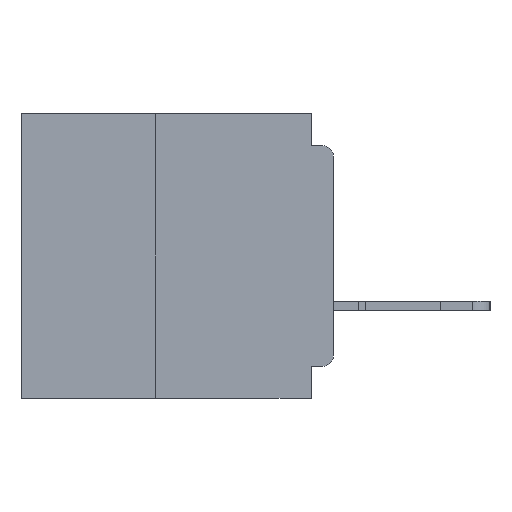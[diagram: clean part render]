
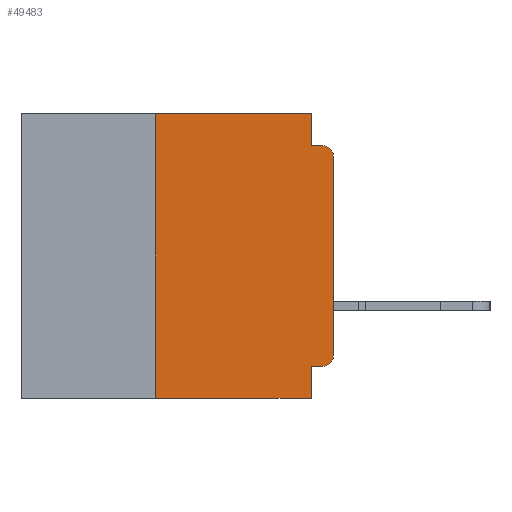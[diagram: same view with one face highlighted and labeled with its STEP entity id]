
A CAD part, left-side view. The second image highlights one B-rep face of the part: STEP entity #49483.
In plain terms, the highlighted planar face has unit normal (-1, 0, 0).
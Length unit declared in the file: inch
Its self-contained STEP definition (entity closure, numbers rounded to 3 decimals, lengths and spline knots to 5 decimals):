
#467 = DIRECTION ( 'NONE',  ( 0., 1., 0. ) ) ;
#2096 = CARTESIAN_POINT ( 'NONE',  ( 0., 0.25, -0.4 ) ) ;
#3207 = EDGE_LOOP ( 'NONE', ( #60867, #43556, #61168, #53774, #62017, #53021, #16379, #43665, #39169, #30989 ) ) ;
#4250 = VECTOR ( 'NONE', #64130, 39.37008 ) ;
#5299 = VERTEX_POINT ( 'NONE', #43062 ) ;
#7291 = LINE ( 'NONE', #30291, #57075 ) ;
#7347 = DIRECTION ( 'NONE',  ( 0., 0., -1. ) ) ;
#8504 = DIRECTION ( 'NONE',  ( 0., -1., 0. ) ) ;
#10152 = CARTESIAN_POINT ( 'NONE',  ( 0., 0.031, 0. ) ) ;
#11619 = EDGE_CURVE ( 'NONE', #15801, #20066, #23603, .T. ) ;
#11772 = VERTEX_POINT ( 'NONE', #50795 ) ;
#12141 = DIRECTION ( 'NONE',  ( 0., 0., 1. ) ) ;
#15801 = VERTEX_POINT ( 'NONE', #27613 ) ;
#15934 = VECTOR ( 'NONE', #12141, 39.37008 ) ;
#16250 = VECTOR ( 'NONE', #8504, 39.37008 ) ;
#16379 = ORIENTED_EDGE ( 'NONE', *, *, #63830, .T. ) ;
#17343 = VERTEX_POINT ( 'NONE', #45705 ) ;
#17473 = LINE ( 'NONE', #39353, #4250 ) ;
#18425 = VERTEX_POINT ( 'NONE', #45819 ) ;
#20066 = VERTEX_POINT ( 'NONE', #33617 ) ;
#20998 = CARTESIAN_POINT ( 'NONE',  ( 0., 0.437, -0.4 ) ) ;
#22725 = AXIS2_PLACEMENT_3D ( 'NONE', #27861, #62647, #32785 ) ;
#23264 = CARTESIAN_POINT ( 'NONE',  ( 0., 0.031, -0.045 ) ) ;
#23603 = CIRCLE ( 'NONE', #56168, 0.015 ) ;
#24756 = CARTESIAN_POINT ( 'NONE',  ( 0., 0.015, -0.34 ) ) ;
#24995 = CIRCLE ( 'NONE', #22725, 0.015 ) ;
#26545 = CARTESIAN_POINT ( 'NONE',  ( 0., 0.031, -0.355 ) ) ;
#27168 = VECTOR ( 'NONE', #44090, 39.37008 ) ;
#27613 = CARTESIAN_POINT ( 'NONE',  ( 0., 0.015, -0.355 ) ) ;
#27861 = CARTESIAN_POINT ( 'NONE',  ( 0., 0.015, -0.06 ) ) ;
#28061 = VERTEX_POINT ( 'NONE', #33551 ) ;
#28755 = LINE ( 'NONE', #39051, #27168 ) ;
#29132 = LINE ( 'NONE', #2096, #15934 ) ;
#29437 = LINE ( 'NONE', #58059, #16250 ) ;
#29734 = DIRECTION ( 'NONE',  ( 0., 0., -1. ) ) ;
#30251 = VERTEX_POINT ( 'NONE', #26545 ) ;
#30272 = VECTOR ( 'NONE', #63655, 39.37008 ) ;
#30291 = CARTESIAN_POINT ( 'NONE',  ( 0., 0., -0.355 ) ) ;
#30989 = ORIENTED_EDGE ( 'NONE', *, *, #11619, .T. ) ;
#31781 = LINE ( 'NONE', #33842, #30272 ) ;
#31805 = EDGE_CURVE ( 'NONE', #18425, #41797, #55300, .T. ) ;
#32033 = PLANE ( 'NONE',  #38515 ) ;
#32785 = DIRECTION ( 'NONE',  ( 0., 0., -1. ) ) ;
#33272 = VERTEX_POINT ( 'NONE', #47868 ) ;
#33551 = CARTESIAN_POINT ( 'NONE',  ( 0., 0.25, 0. ) ) ;
#33617 = CARTESIAN_POINT ( 'NONE',  ( 0., 0., -0.34 ) ) ;
#33842 = CARTESIAN_POINT ( 'NONE',  ( 0., 0.031, -0.4 ) ) ;
#35235 = DIRECTION ( 'NONE',  ( 0., 0., -1. ) ) ;
#36512 = EDGE_CURVE ( 'NONE', #15801, #30251, #7291, .T. ) ;
#37047 = DIRECTION ( 'NONE',  ( 1., 0., 0. ) ) ;
#38515 = AXIS2_PLACEMENT_3D ( 'NONE', #56709, #37047, #7347 ) ;
#39051 = CARTESIAN_POINT ( 'NONE',  ( 0., 0., 0. ) ) ;
#39169 = ORIENTED_EDGE ( 'NONE', *, *, #36512, .F. ) ;
#39353 = CARTESIAN_POINT ( 'NONE',  ( 0., 0.437, 0. ) ) ;
#41797 = VERTEX_POINT ( 'NONE', #23264 ) ;
#41798 = EDGE_CURVE ( 'NONE', #41797, #5299, #29437, .T. ) ;
#42039 = VECTOR ( 'NONE', #35235, 39.37008 ) ;
#43062 = CARTESIAN_POINT ( 'NONE',  ( 0., 0.015, -0.045 ) ) ;
#43556 = ORIENTED_EDGE ( 'NONE', *, *, #59804, .T. ) ;
#43665 = ORIENTED_EDGE ( 'NONE', *, *, #60733, .F. ) ;
#44090 = DIRECTION ( 'NONE',  ( 0., 0., 1. ) ) ;
#44157 = FACE_OUTER_BOUND ( 'NONE', #3207, .T. ) ;
#45705 = CARTESIAN_POINT ( 'NONE',  ( 0., 0., -0.06 ) ) ;
#45819 = CARTESIAN_POINT ( 'NONE',  ( 0., 0.031, 0. ) ) ;
#47868 = CARTESIAN_POINT ( 'NONE',  ( 0., 0.031, -0.4 ) ) ;
#49483 = ADVANCED_FACE ( 'NONE', ( #44157 ), #32033, .F. ) ;
#50795 = CARTESIAN_POINT ( 'NONE',  ( 0., 0.25, -0.4 ) ) ;
#51195 = EDGE_CURVE ( 'NONE', #11772, #28061, #29132, .T. ) ;
#53021 = ORIENTED_EDGE ( 'NONE', *, *, #51195, .F. ) ;
#53774 = ORIENTED_EDGE ( 'NONE', *, *, #31805, .F. ) ;
#53869 = EDGE_CURVE ( 'NONE', #20066, #17343, #28755, .T. ) ;
#55300 = LINE ( 'NONE', #10152, #42039 ) ;
#56168 = AXIS2_PLACEMENT_3D ( 'NONE', #24756, #59527, #29734 ) ;
#56709 = CARTESIAN_POINT ( 'NONE',  ( 0., 0.437, 0. ) ) ;
#57075 = VECTOR ( 'NONE', #467, 39.37008 ) ;
#58059 = CARTESIAN_POINT ( 'NONE',  ( 0., 0., -0.045 ) ) ;
#58184 = EDGE_CURVE ( 'NONE', #28061, #18425, #17473, .T. ) ;
#59410 = LINE ( 'NONE', #20998, #60962 ) ;
#59527 = DIRECTION ( 'NONE',  ( -1., 0., 0. ) ) ;
#59804 = EDGE_CURVE ( 'NONE', #17343, #5299, #24995, .T. ) ;
#60733 = EDGE_CURVE ( 'NONE', #30251, #33272, #31781, .T. ) ;
#60765 = DIRECTION ( 'NONE',  ( 0., -1., 0. ) ) ;
#60867 = ORIENTED_EDGE ( 'NONE', *, *, #53869, .T. ) ;
#60962 = VECTOR ( 'NONE', #60765, 39.37008 ) ;
#61168 = ORIENTED_EDGE ( 'NONE', *, *, #41798, .F. ) ;
#62017 = ORIENTED_EDGE ( 'NONE', *, *, #58184, .F. ) ;
#62647 = DIRECTION ( 'NONE',  ( -1., 0., 0. ) ) ;
#63655 = DIRECTION ( 'NONE',  ( 0., 0., -1. ) ) ;
#63830 = EDGE_CURVE ( 'NONE', #11772, #33272, #59410, .T. ) ;
#64130 = DIRECTION ( 'NONE',  ( 0., -1., 0. ) ) ;
